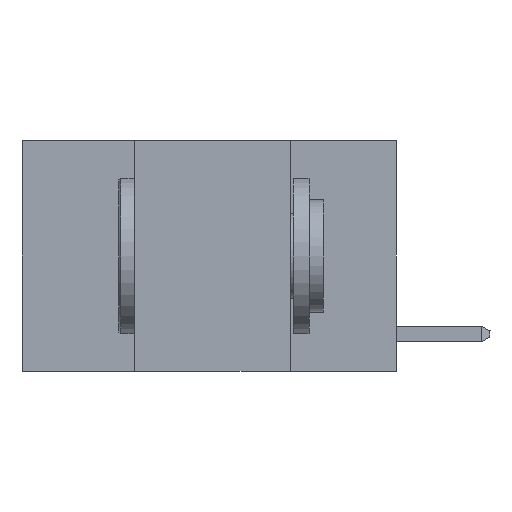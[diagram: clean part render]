
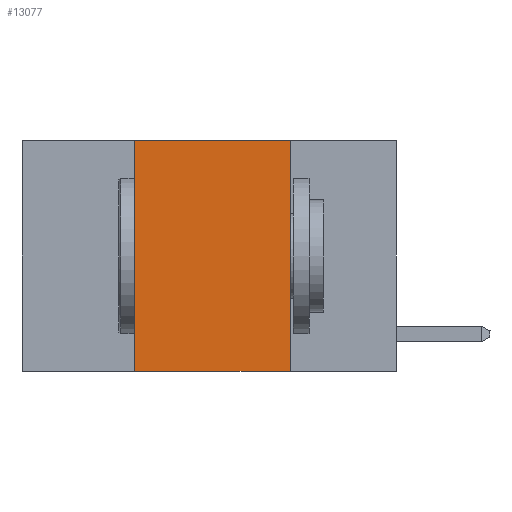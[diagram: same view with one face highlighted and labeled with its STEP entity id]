
A CAD part, left-side view. The second image highlights one B-rep face of the part: STEP entity #13077.
In plain terms, the highlighted planar face has unit normal (-1, 0, 0).
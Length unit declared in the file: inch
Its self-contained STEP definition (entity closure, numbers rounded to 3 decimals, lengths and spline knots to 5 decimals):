
#537 = LINE ( 'NONE', #5288, #8684 ) ;
#797 = EDGE_CURVE ( 'NONE', #1245, #12510, #537, .T. ) ;
#876 = EDGE_CURVE ( 'NONE', #7180, #2458, #7044, .T. ) ;
#1060 = DIRECTION ( 'NONE',  ( 0., 0., 1. ) ) ;
#1245 = VERTEX_POINT ( 'NONE', #10511 ) ;
#1844 = ORIENTED_EDGE ( 'NONE', *, *, #3968, .T. ) ;
#2458 = VERTEX_POINT ( 'NONE', #9306 ) ;
#2677 = FACE_OUTER_BOUND ( 'NONE', #7296, .T. ) ;
#3062 = EDGE_CURVE ( 'NONE', #12510, #7180, #3892, .T. ) ;
#3214 = VECTOR ( 'NONE', #12076, 39.37008 ) ;
#3299 = DIRECTION ( 'NONE',  ( 0., -1., 0. ) ) ;
#3892 = LINE ( 'NONE', #8750, #3214 ) ;
#3968 = EDGE_CURVE ( 'NONE', #1245, #2458, #5861, .T. ) ;
#4528 = CARTESIAN_POINT ( 'NONE',  ( 0., 0.6, 0. ) ) ;
#5288 = CARTESIAN_POINT ( 'NONE',  ( 0., 0.42, 0. ) ) ;
#5396 = CARTESIAN_POINT ( 'NONE',  ( 0., 0.6, -0.37 ) ) ;
#5861 = LINE ( 'NONE', #5396, #8028 ) ;
#6363 = AXIS2_PLACEMENT_3D ( 'NONE', #4528, #12886, #9728 ) ;
#7044 = LINE ( 'NONE', #10033, #8526 ) ;
#7180 = VERTEX_POINT ( 'NONE', #9888 ) ;
#7296 = EDGE_LOOP ( 'NONE', ( #8511, #9500, #13037, #1844 ) ) ;
#7698 = PLANE ( 'NONE',  #6363 ) ;
#8028 = VECTOR ( 'NONE', #3299, 39.37008 ) ;
#8511 = ORIENTED_EDGE ( 'NONE', *, *, #876, .F. ) ;
#8526 = VECTOR ( 'NONE', #9514, 39.37008 ) ;
#8684 = VECTOR ( 'NONE', #1060, 39.37008 ) ;
#8750 = CARTESIAN_POINT ( 'NONE',  ( 0., 0.6, 0. ) ) ;
#8804 = CARTESIAN_POINT ( 'NONE',  ( 0., 0.42, 0. ) ) ;
#9306 = CARTESIAN_POINT ( 'NONE',  ( 0., 0.17, -0.37 ) ) ;
#9500 = ORIENTED_EDGE ( 'NONE', *, *, #3062, .F. ) ;
#9514 = DIRECTION ( 'NONE',  ( 0., 0., -1. ) ) ;
#9728 = DIRECTION ( 'NONE',  ( 0., 0., -1. ) ) ;
#9888 = CARTESIAN_POINT ( 'NONE',  ( 0., 0.17, 0. ) ) ;
#10033 = CARTESIAN_POINT ( 'NONE',  ( 0., 0.17, 0. ) ) ;
#10511 = CARTESIAN_POINT ( 'NONE',  ( 0., 0.42, -0.37 ) ) ;
#12076 = DIRECTION ( 'NONE',  ( 0., -1., 0. ) ) ;
#12510 = VERTEX_POINT ( 'NONE', #8804 ) ;
#12886 = DIRECTION ( 'NONE',  ( 1., 0., 0. ) ) ;
#13037 = ORIENTED_EDGE ( 'NONE', *, *, #797, .F. ) ;
#13077 = ADVANCED_FACE ( 'NONE', ( #2677 ), #7698, .F. ) ;
